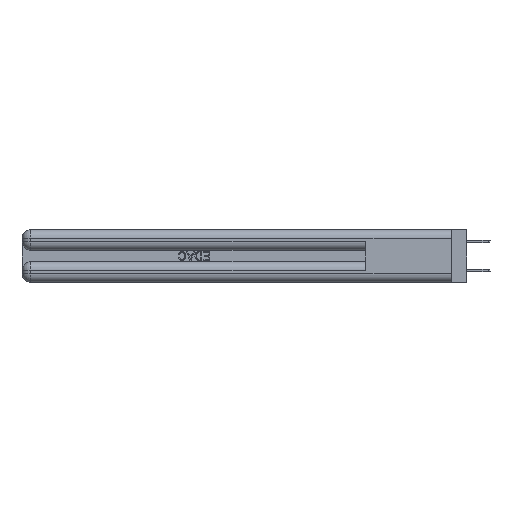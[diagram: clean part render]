
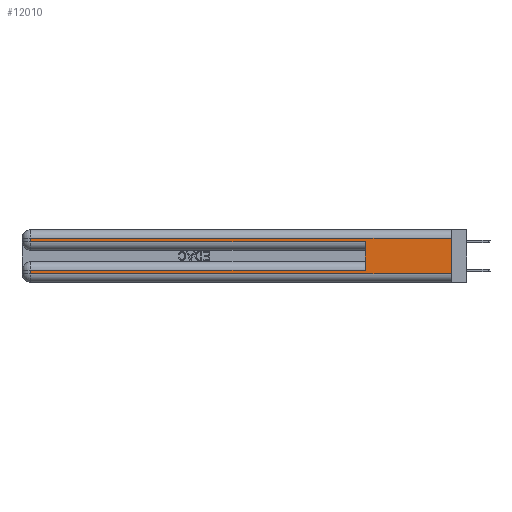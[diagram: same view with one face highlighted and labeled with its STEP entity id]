
A CAD part, left-side view. The second image highlights one B-rep face of the part: STEP entity #12010.
In plain terms, the highlighted planar face has unit normal (-1, 0, 0).
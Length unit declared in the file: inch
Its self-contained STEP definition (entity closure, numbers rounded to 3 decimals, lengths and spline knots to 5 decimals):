
#105 = EDGE_CURVE ( 'NONE', #5384, #22717, #7023, .T. ) ;
#342 = VERTEX_POINT ( 'NONE', #36484 ) ;
#1299 = LINE ( 'NONE', #39069, #26316 ) ;
#3633 = CARTESIAN_POINT ( 'NONE',  ( 0., 0.6, 0.145 ) ) ;
#4871 = DIRECTION ( 'NONE',  ( 0., 1., 0. ) ) ;
#5384 = VERTEX_POINT ( 'NONE', #10712 ) ;
#7023 = LINE ( 'NONE', #19086, #23423 ) ;
#7143 = CARTESIAN_POINT ( 'NONE',  ( 0., 0.6, 0.285 ) ) ;
#8776 = VERTEX_POINT ( 'NONE', #17376 ) ;
#8881 = CARTESIAN_POINT ( 'NONE',  ( 0., 0.6, 0.085 ) ) ;
#8962 = ORIENTED_EDGE ( 'NONE', *, *, #13282, .T. ) ;
#9143 = ORIENTED_EDGE ( 'NONE', *, *, #18228, .F. ) ;
#9614 = DIRECTION ( 'NONE',  ( 0., 1., 0. ) ) ;
#10024 = ORIENTED_EDGE ( 'NONE', *, *, #105, .T. ) ;
#10343 = EDGE_CURVE ( 'NONE', #8776, #23347, #23807, .T. ) ;
#10712 = CARTESIAN_POINT ( 'NONE',  ( 0., 2.94, 0.06 ) ) ;
#11033 = ORIENTED_EDGE ( 'NONE', *, *, #10343, .T. ) ;
#11112 = ORIENTED_EDGE ( 'NONE', *, *, #16674, .T. ) ;
#11763 = DIRECTION ( 'NONE',  ( 0., 0., -1. ) ) ;
#12010 = ADVANCED_FACE ( 'NONE', ( #21119 ), #40655, .F. ) ;
#12479 = EDGE_LOOP ( 'NONE', ( #38937, #8962, #11033, #23913, #9143, #39997, #11112, #10024 ) ) ;
#13120 = VECTOR ( 'NONE', #23193, 39.37008 ) ;
#13282 = EDGE_CURVE ( 'NONE', #22804, #8776, #17430, .T. ) ;
#13683 = LINE ( 'NONE', #26281, #38728 ) ;
#16454 = CARTESIAN_POINT ( 'NONE',  ( 0., 0., 0.31 ) ) ;
#16674 = EDGE_CURVE ( 'NONE', #342, #5384, #36288, .T. ) ;
#17376 = CARTESIAN_POINT ( 'NONE',  ( 0., 2.94, 0.31 ) ) ;
#17430 = LINE ( 'NONE', #34297, #25082 ) ;
#17954 = DIRECTION ( 'NONE',  ( 0., 0., -1. ) ) ;
#18228 = EDGE_CURVE ( 'NONE', #20154, #22926, #21841, .T. ) ;
#19086 = CARTESIAN_POINT ( 'NONE',  ( 0., 0., 0.06 ) ) ;
#19660 = EDGE_CURVE ( 'NONE', #20154, #342, #1299, .T. ) ;
#20154 = VERTEX_POINT ( 'NONE', #8881 ) ;
#21119 = FACE_OUTER_BOUND ( 'NONE', #12479, .T. ) ;
#21841 = LINE ( 'NONE', #3633, #13120 ) ;
#22037 = CARTESIAN_POINT ( 'NONE',  ( 0., 2.94, 0.37 ) ) ;
#22717 = VERTEX_POINT ( 'NONE', #32367 ) ;
#22804 = VERTEX_POINT ( 'NONE', #16454 ) ;
#22926 = VERTEX_POINT ( 'NONE', #7143 ) ;
#23193 = DIRECTION ( 'NONE',  ( 0., 0., 1. ) ) ;
#23347 = VERTEX_POINT ( 'NONE', #35300 ) ;
#23423 = VECTOR ( 'NONE', #41914, 39.37008 ) ;
#23807 = LINE ( 'NONE', #34653, #40169 ) ;
#23913 = ORIENTED_EDGE ( 'NONE', *, *, #24950, .T. ) ;
#24950 = EDGE_CURVE ( 'NONE', #23347, #22926, #13683, .T. ) ;
#25082 = VECTOR ( 'NONE', #4871, 39.37008 ) ;
#25336 = CARTESIAN_POINT ( 'NONE',  ( 0., 0., 0.37 ) ) ;
#26281 = CARTESIAN_POINT ( 'NONE',  ( 0., 0., 0.285 ) ) ;
#26316 = VECTOR ( 'NONE', #9614, 39.37008 ) ;
#27039 = VECTOR ( 'NONE', #31941, 39.37008 ) ;
#27618 = VECTOR ( 'NONE', #41742, 39.37008 ) ;
#27665 = CARTESIAN_POINT ( 'NONE',  ( 0., 0., 0.37 ) ) ;
#31941 = DIRECTION ( 'NONE',  ( 0., 0., -1. ) ) ;
#32367 = CARTESIAN_POINT ( 'NONE',  ( 0., 0., 0.06 ) ) ;
#32777 = EDGE_CURVE ( 'NONE', #22804, #22717, #34699, .T. ) ;
#34297 = CARTESIAN_POINT ( 'NONE',  ( 0., 0., 0.31 ) ) ;
#34653 = CARTESIAN_POINT ( 'NONE',  ( 0., 2.94, 0.37 ) ) ;
#34699 = LINE ( 'NONE', #25336, #27039 ) ;
#35300 = CARTESIAN_POINT ( 'NONE',  ( 0., 2.94, 0.285 ) ) ;
#36288 = LINE ( 'NONE', #22037, #27618 ) ;
#36484 = CARTESIAN_POINT ( 'NONE',  ( 0., 2.94, 0.085 ) ) ;
#37512 = DIRECTION ( 'NONE',  ( 1., 0., 0. ) ) ;
#38209 = AXIS2_PLACEMENT_3D ( 'NONE', #27665, #37512, #17954 ) ;
#38728 = VECTOR ( 'NONE', #39247, 39.37008 ) ;
#38937 = ORIENTED_EDGE ( 'NONE', *, *, #32777, .F. ) ;
#39069 = CARTESIAN_POINT ( 'NONE',  ( 0., 0., 0.085 ) ) ;
#39247 = DIRECTION ( 'NONE',  ( 0., -1., 0. ) ) ;
#39997 = ORIENTED_EDGE ( 'NONE', *, *, #19660, .T. ) ;
#40169 = VECTOR ( 'NONE', #11763, 39.37008 ) ;
#40655 = PLANE ( 'NONE',  #38209 ) ;
#41742 = DIRECTION ( 'NONE',  ( 0., 0., -1. ) ) ;
#41914 = DIRECTION ( 'NONE',  ( 0., -1., 0. ) ) ;
